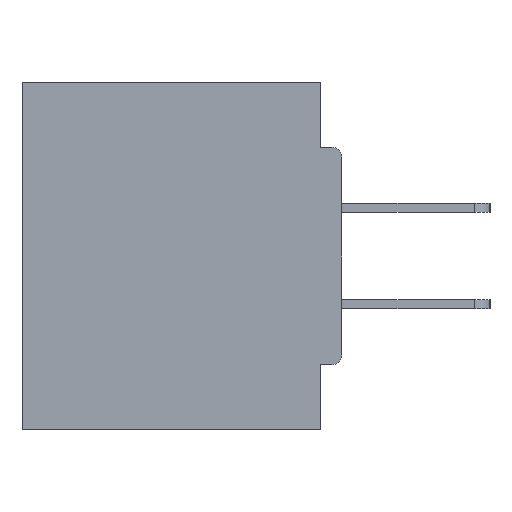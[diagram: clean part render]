
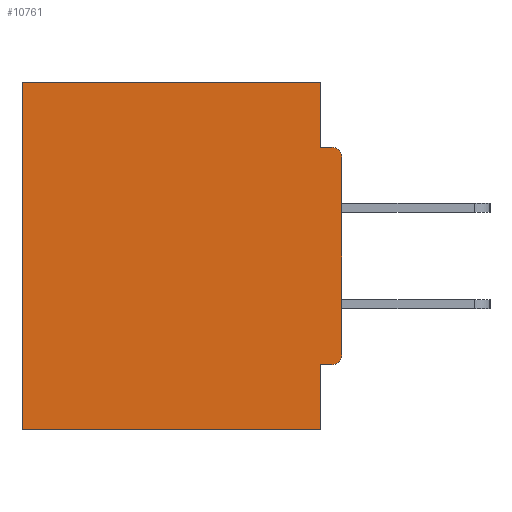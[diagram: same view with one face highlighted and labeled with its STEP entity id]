
A CAD part, left-side view. The second image highlights one B-rep face of the part: STEP entity #10761.
In plain terms, the highlighted planar face has unit normal (-1, 0, 0).
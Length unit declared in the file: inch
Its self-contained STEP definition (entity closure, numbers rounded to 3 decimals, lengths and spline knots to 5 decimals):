
#771 = AXIS2_PLACEMENT_3D ( 'NONE', #7150, #3966, #12707 ) ;
#1956 = LINE ( 'NONE', #28158, #9731 ) ;
#2560 = DIRECTION ( 'NONE',  ( 0., 0., -1. ) ) ;
#3877 = LINE ( 'NONE', #31200, #33481 ) ;
#3888 = CIRCLE ( 'NONE', #771, 0.015 ) ;
#3966 = DIRECTION ( 'NONE',  ( -1., 0., 0. ) ) ;
#4127 = EDGE_LOOP ( 'NONE', ( #28413, #35571, #13006, #32331, #21117, #22573, #36368, #23883, #6345, #14291 ) ) ;
#4447 = CARTESIAN_POINT ( 'NONE',  ( 0.298, 0.015, -0.4065 ) ) ;
#4849 = CARTESIAN_POINT ( 'NONE',  ( 0.298, 0., 0. ) ) ;
#5460 = EDGE_CURVE ( 'NONE', #17480, #11312, #10113, .T. ) ;
#5707 = LINE ( 'NONE', #12800, #26971 ) ;
#6345 = ORIENTED_EDGE ( 'NONE', *, *, #24054, .T. ) ;
#6439 = EDGE_CURVE ( 'NONE', #9737, #17480, #14719, .T. ) ;
#6859 = DIRECTION ( 'NONE',  ( 0., 1., 0. ) ) ;
#7150 = CARTESIAN_POINT ( 'NONE',  ( 0.298, 0.015, -0.3915 ) ) ;
#7810 = DIRECTION ( 'NONE',  ( 0., 1., 0. ) ) ;
#8180 = CARTESIAN_POINT ( 'NONE',  ( 0.298, 0., -0.3915 ) ) ;
#8692 = CARTESIAN_POINT ( 'NONE',  ( 0.298, 0.031, -0.0935 ) ) ;
#8778 = LINE ( 'NONE', #29473, #37535 ) ;
#9448 = VERTEX_POINT ( 'NONE', #10160 ) ;
#9667 = EDGE_CURVE ( 'NONE', #11295, #9448, #3877, .T. ) ;
#9718 = FACE_OUTER_BOUND ( 'NONE', #4127, .T. ) ;
#9731 = VECTOR ( 'NONE', #37386, 39.37008 ) ;
#9737 = VERTEX_POINT ( 'NONE', #4447 ) ;
#10113 = LINE ( 'NONE', #26726, #32344 ) ;
#10160 = CARTESIAN_POINT ( 'NONE',  ( 0.298, 0.015, -0.0935 ) ) ;
#10170 = LINE ( 'NONE', #4849, #19395 ) ;
#10297 = DIRECTION ( 'NONE',  ( 1., 0., 0. ) ) ;
#10680 = VERTEX_POINT ( 'NONE', #30615 ) ;
#10761 = ADVANCED_FACE ( 'NONE', ( #9718 ), #13132, .F. ) ;
#11208 = EDGE_CURVE ( 'NONE', #12170, #28014, #10170, .T. ) ;
#11295 = VERTEX_POINT ( 'NONE', #8692 ) ;
#11312 = VERTEX_POINT ( 'NONE', #23279 ) ;
#11583 = AXIS2_PLACEMENT_3D ( 'NONE', #20165, #32486, #2560 ) ;
#12126 = CIRCLE ( 'NONE', #11583, 0.015 ) ;
#12170 = VERTEX_POINT ( 'NONE', #13737 ) ;
#12707 = DIRECTION ( 'NONE',  ( 0., 0., -1. ) ) ;
#12800 = CARTESIAN_POINT ( 'NONE',  ( 0.298, 0., -0.5 ) ) ;
#13006 = ORIENTED_EDGE ( 'NONE', *, *, #25713, .F. ) ;
#13132 = PLANE ( 'NONE',  #21580 ) ;
#13506 = DIRECTION ( 'NONE',  ( 0., 0., -1. ) ) ;
#13582 = CARTESIAN_POINT ( 'NONE',  ( 0.298, 0., -0.4065 ) ) ;
#13737 = CARTESIAN_POINT ( 'NONE',  ( 0.298, 0.031, 0. ) ) ;
#14291 = ORIENTED_EDGE ( 'NONE', *, *, #25249, .F. ) ;
#14719 = LINE ( 'NONE', #13582, #22545 ) ;
#14819 = DIRECTION ( 'NONE',  ( 0., 0., -1. ) ) ;
#16147 = DIRECTION ( 'NONE',  ( 0., -1., 0. ) ) ;
#16562 = VERTEX_POINT ( 'NONE', #8180 ) ;
#17480 = VERTEX_POINT ( 'NONE', #20287 ) ;
#17528 = VERTEX_POINT ( 'NONE', #26497 ) ;
#17829 = DIRECTION ( 'NONE',  ( 0., 0., -1. ) ) ;
#19395 = VECTOR ( 'NONE', #7810, 39.37008 ) ;
#20165 = CARTESIAN_POINT ( 'NONE',  ( 0.298, 0.015, -0.1085 ) ) ;
#20287 = CARTESIAN_POINT ( 'NONE',  ( 0.298, 0.031, -0.4065 ) ) ;
#21117 = ORIENTED_EDGE ( 'NONE', *, *, #28397, .T. ) ;
#21474 = EDGE_CURVE ( 'NONE', #11312, #10680, #5707, .T. ) ;
#21580 = AXIS2_PLACEMENT_3D ( 'NONE', #37118, #10297, #13506 ) ;
#22545 = VECTOR ( 'NONE', #33814, 39.37008 ) ;
#22573 = ORIENTED_EDGE ( 'NONE', *, *, #21474, .F. ) ;
#23097 = CARTESIAN_POINT ( 'NONE',  ( 0.298, 0.46, 0. ) ) ;
#23279 = CARTESIAN_POINT ( 'NONE',  ( 0.298, 0.031, -0.5 ) ) ;
#23883 = ORIENTED_EDGE ( 'NONE', *, *, #6439, .F. ) ;
#24054 = EDGE_CURVE ( 'NONE', #9737, #16562, #3888, .T. ) ;
#25249 = EDGE_CURVE ( 'NONE', #17528, #16562, #1956, .T. ) ;
#25713 = EDGE_CURVE ( 'NONE', #12170, #11295, #8778, .T. ) ;
#26497 = CARTESIAN_POINT ( 'NONE',  ( 0.298, 0., -0.1085 ) ) ;
#26726 = CARTESIAN_POINT ( 'NONE',  ( 0.298, 0.031, -0.5 ) ) ;
#26971 = VECTOR ( 'NONE', #6859, 39.37008 ) ;
#27119 = VECTOR ( 'NONE', #17829, 39.37008 ) ;
#28014 = VERTEX_POINT ( 'NONE', #23097 ) ;
#28158 = CARTESIAN_POINT ( 'NONE',  ( 0.298, 0., 0. ) ) ;
#28397 = EDGE_CURVE ( 'NONE', #28014, #10680, #28996, .T. ) ;
#28413 = ORIENTED_EDGE ( 'NONE', *, *, #32690, .T. ) ;
#28996 = LINE ( 'NONE', #29491, #27119 ) ;
#29473 = CARTESIAN_POINT ( 'NONE',  ( 0.298, 0.031, -0.5 ) ) ;
#29491 = CARTESIAN_POINT ( 'NONE',  ( 0.298, 0.46, 0. ) ) ;
#30615 = CARTESIAN_POINT ( 'NONE',  ( 0.298, 0.46, -0.5 ) ) ;
#31200 = CARTESIAN_POINT ( 'NONE',  ( 0.298, 0., -0.0935 ) ) ;
#32331 = ORIENTED_EDGE ( 'NONE', *, *, #11208, .T. ) ;
#32344 = VECTOR ( 'NONE', #14819, 39.37008 ) ;
#32486 = DIRECTION ( 'NONE',  ( -1., 0., 0. ) ) ;
#32690 = EDGE_CURVE ( 'NONE', #17528, #9448, #12126, .T. ) ;
#33481 = VECTOR ( 'NONE', #16147, 39.37008 ) ;
#33814 = DIRECTION ( 'NONE',  ( 0., 1., 0. ) ) ;
#35571 = ORIENTED_EDGE ( 'NONE', *, *, #9667, .F. ) ;
#36368 = ORIENTED_EDGE ( 'NONE', *, *, #5460, .F. ) ;
#37118 = CARTESIAN_POINT ( 'NONE',  ( 0.298, 0., 0. ) ) ;
#37386 = DIRECTION ( 'NONE',  ( 0., 0., -1. ) ) ;
#37535 = VECTOR ( 'NONE', #38231, 39.37008 ) ;
#38231 = DIRECTION ( 'NONE',  ( 0., 0., -1. ) ) ;
